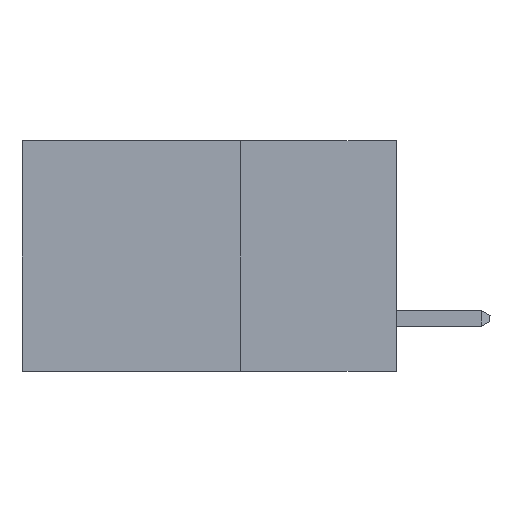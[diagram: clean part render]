
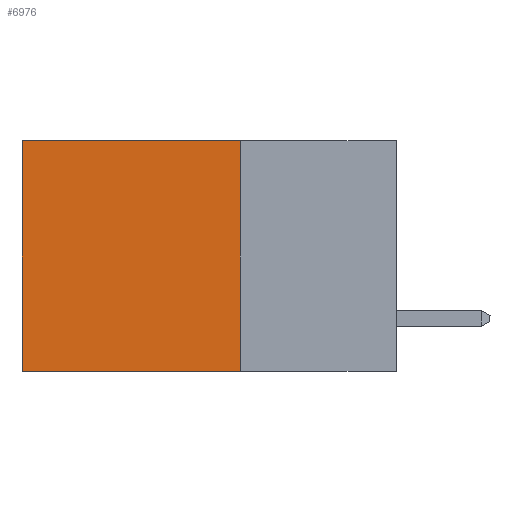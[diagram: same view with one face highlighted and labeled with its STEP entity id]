
A CAD part, left-side view. The second image highlights one B-rep face of the part: STEP entity #6976.
In plain terms, the highlighted planar face has unit normal (-1, 0, 0).
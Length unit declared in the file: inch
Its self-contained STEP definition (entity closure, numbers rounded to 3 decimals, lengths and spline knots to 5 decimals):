
#195 = EDGE_CURVE ( 'NONE', #15522, #6096, #14295, .T. ) ;
#309 = AXIS2_PLACEMENT_3D ( 'NONE', #11748, #2271, #13389 ) ;
#1055 = ORIENTED_EDGE ( 'NONE', *, *, #18030, .T. ) ;
#1351 = VECTOR ( 'NONE', #18264, 39.37008 ) ;
#2069 = EDGE_LOOP ( 'NONE', ( #1055, #13117, #16968, #11458 ) ) ;
#2271 = DIRECTION ( 'NONE',  ( 1., 0., 0. ) ) ;
#2539 = CARTESIAN_POINT ( 'NONE',  ( 0.2615, 0.6, -0.37 ) ) ;
#3627 = LINE ( 'NONE', #13252, #7371 ) ;
#3790 = PLANE ( 'NONE',  #309 ) ;
#5091 = CARTESIAN_POINT ( 'NONE',  ( 0.2615, 0.6, -0.37 ) ) ;
#5153 = EDGE_CURVE ( 'NONE', #13132, #15522, #3627, .T. ) ;
#5801 = VECTOR ( 'NONE', #17269, 39.37008 ) ;
#6096 = VERTEX_POINT ( 'NONE', #5091 ) ;
#6976 = ADVANCED_FACE ( 'NONE', ( #12342 ), #3790, .F. ) ;
#7371 = VECTOR ( 'NONE', #13319, 39.37008 ) ;
#8451 = CARTESIAN_POINT ( 'NONE',  ( 0.2615, 0.25, -0.37 ) ) ;
#8771 = CARTESIAN_POINT ( 'NONE',  ( 0.2615, 0.25, 0. ) ) ;
#10421 = DIRECTION ( 'NONE',  ( 0., 0., -1. ) ) ;
#11458 = ORIENTED_EDGE ( 'NONE', *, *, #18985, .T. ) ;
#11748 = CARTESIAN_POINT ( 'NONE',  ( 0.2615, 0.25, -0.37 ) ) ;
#12342 = FACE_OUTER_BOUND ( 'NONE', #2069, .T. ) ;
#13117 = ORIENTED_EDGE ( 'NONE', *, *, #195, .F. ) ;
#13132 = VERTEX_POINT ( 'NONE', #19933 ) ;
#13252 = CARTESIAN_POINT ( 'NONE',  ( 0.2615, 0.25, -0.37 ) ) ;
#13319 = DIRECTION ( 'NONE',  ( 0., 0., -1. ) ) ;
#13389 = DIRECTION ( 'NONE',  ( 0., 0., -1. ) ) ;
#13597 = CARTESIAN_POINT ( 'NONE',  ( 0.2615, 0.6, 0. ) ) ;
#14295 = LINE ( 'NONE', #16819, #5801 ) ;
#14352 = VERTEX_POINT ( 'NONE', #13597 ) ;
#15522 = VERTEX_POINT ( 'NONE', #8451 ) ;
#16527 = VECTOR ( 'NONE', #10421, 39.37008 ) ;
#16819 = CARTESIAN_POINT ( 'NONE',  ( 0.2615, 0.25, -0.37 ) ) ;
#16968 = ORIENTED_EDGE ( 'NONE', *, *, #5153, .F. ) ;
#17015 = LINE ( 'NONE', #2539, #16527 ) ;
#17269 = DIRECTION ( 'NONE',  ( 0., 1., 0. ) ) ;
#18030 = EDGE_CURVE ( 'NONE', #14352, #6096, #17015, .T. ) ;
#18264 = DIRECTION ( 'NONE',  ( 0., 1., 0. ) ) ;
#18666 = LINE ( 'NONE', #8771, #1351 ) ;
#18985 = EDGE_CURVE ( 'NONE', #13132, #14352, #18666, .T. ) ;
#19933 = CARTESIAN_POINT ( 'NONE',  ( 0.2615, 0.25, 0. ) ) ;
